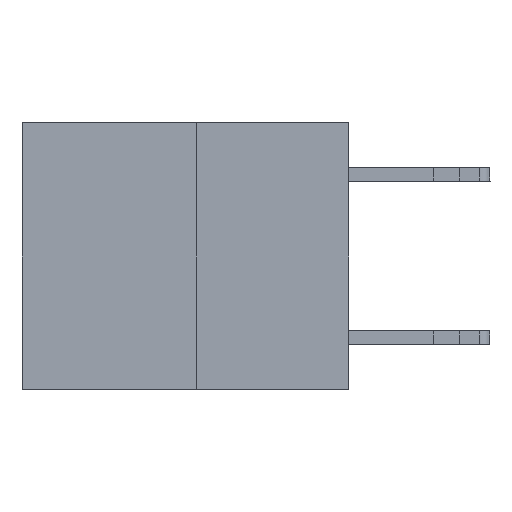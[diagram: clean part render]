
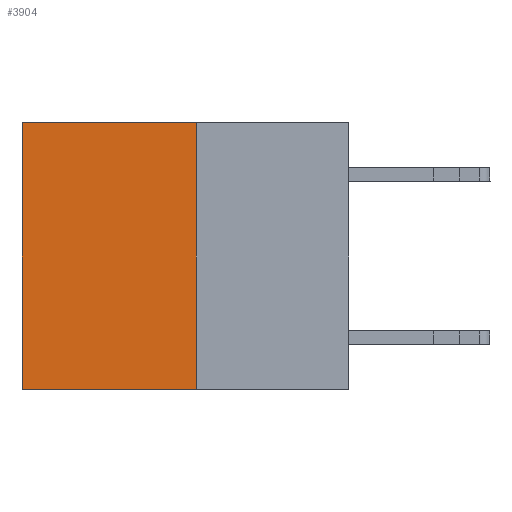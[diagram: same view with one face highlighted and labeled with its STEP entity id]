
A CAD part, left-side view. The second image highlights one B-rep face of the part: STEP entity #3904.
In plain terms, the highlighted planar face has unit normal (-1, 0, 0).
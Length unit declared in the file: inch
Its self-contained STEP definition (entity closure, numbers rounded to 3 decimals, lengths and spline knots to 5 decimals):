
#432 = CARTESIAN_POINT ( 'NONE',  ( 0.3165, 0.6, -0.49 ) ) ;
#3010 = EDGE_CURVE ( 'NONE', #6919, #5911, #17448, .T. ) ;
#3144 = EDGE_LOOP ( 'NONE', ( #19203, #13456, #15929, #9294 ) ) ;
#3904 = ADVANCED_FACE ( 'NONE', ( #10494 ), #8242, .F. ) ;
#4481 = CARTESIAN_POINT ( 'NONE',  ( 0.3165, 0.28, -0.49 ) ) ;
#5540 = CARTESIAN_POINT ( 'NONE',  ( 0.3165, 0.28, -0.49 ) ) ;
#5875 = EDGE_CURVE ( 'NONE', #6787, #10513, #17668, .T. ) ;
#5911 = VERTEX_POINT ( 'NONE', #14910 ) ;
#6654 = DIRECTION ( 'NONE',  ( 0., 0., -1. ) ) ;
#6710 = DIRECTION ( 'NONE',  ( 0., 0., -1. ) ) ;
#6787 = VERTEX_POINT ( 'NONE', #4481 ) ;
#6919 = VERTEX_POINT ( 'NONE', #13762 ) ;
#7029 = VECTOR ( 'NONE', #9071, 39.37008 ) ;
#7762 = VECTOR ( 'NONE', #13134, 39.37008 ) ;
#7764 = CARTESIAN_POINT ( 'NONE',  ( 0.3165, 0.28, 0. ) ) ;
#8242 = PLANE ( 'NONE',  #8491 ) ;
#8491 = AXIS2_PLACEMENT_3D ( 'NONE', #17222, #20625, #6710 ) ;
#8568 = CARTESIAN_POINT ( 'NONE',  ( 0.3165, 0.6, -0.49 ) ) ;
#9071 = DIRECTION ( 'NONE',  ( 0., 0., -1. ) ) ;
#9294 = ORIENTED_EDGE ( 'NONE', *, *, #3010, .T. ) ;
#9635 = CARTESIAN_POINT ( 'NONE',  ( 0.3165, 0.28, -0.49 ) ) ;
#10494 = FACE_OUTER_BOUND ( 'NONE', #3144, .T. ) ;
#10513 = VERTEX_POINT ( 'NONE', #432 ) ;
#10760 = VECTOR ( 'NONE', #21994, 39.37008 ) ;
#13134 = DIRECTION ( 'NONE',  ( 0., 1., 0. ) ) ;
#13456 = ORIENTED_EDGE ( 'NONE', *, *, #5875, .F. ) ;
#13762 = CARTESIAN_POINT ( 'NONE',  ( 0.3165, 0.28, 0. ) ) ;
#14702 = EDGE_CURVE ( 'NONE', #5911, #10513, #21496, .T. ) ;
#14910 = CARTESIAN_POINT ( 'NONE',  ( 0.3165, 0.6, 0. ) ) ;
#15449 = VECTOR ( 'NONE', #6654, 39.37008 ) ;
#15929 = ORIENTED_EDGE ( 'NONE', *, *, #16810, .F. ) ;
#16810 = EDGE_CURVE ( 'NONE', #6919, #6787, #16980, .T. ) ;
#16980 = LINE ( 'NONE', #5540, #7029 ) ;
#17222 = CARTESIAN_POINT ( 'NONE',  ( 0.3165, 0.28, -0.49 ) ) ;
#17448 = LINE ( 'NONE', #7764, #7762 ) ;
#17668 = LINE ( 'NONE', #9635, #10760 ) ;
#19203 = ORIENTED_EDGE ( 'NONE', *, *, #14702, .T. ) ;
#20625 = DIRECTION ( 'NONE',  ( 1., 0., 0. ) ) ;
#21496 = LINE ( 'NONE', #8568, #15449 ) ;
#21994 = DIRECTION ( 'NONE',  ( 0., 1., 0. ) ) ;
